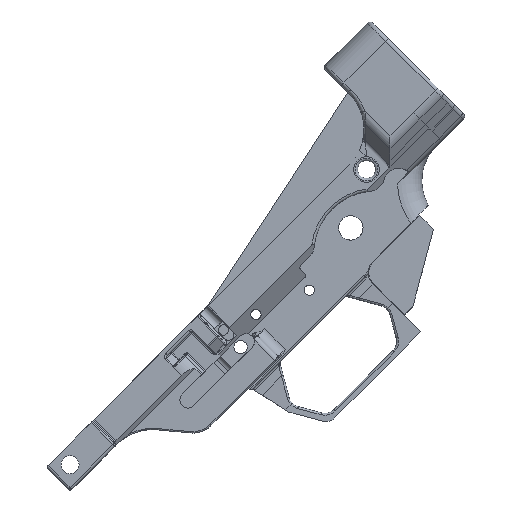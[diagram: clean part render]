
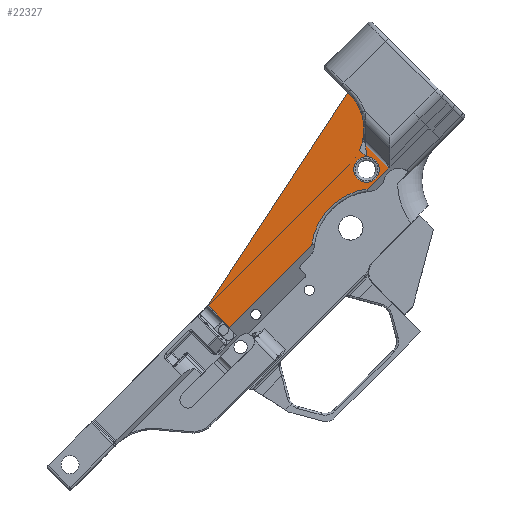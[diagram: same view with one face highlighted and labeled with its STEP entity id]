
A CAD part, front view. The second image highlights one B-rep face of the part: STEP entity #22327.
In plain terms, the highlighted planar face has unit normal (0, -1, 0).
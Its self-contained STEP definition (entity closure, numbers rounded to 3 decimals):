
#5577=CARTESIAN_POINT('',(-25.441,-18.567,22.339));
#5578=VERTEX_POINT('',#5577);
#5586=CARTESIAN_POINT('',(29.722,-18.567,77.502));
#5587=VERTEX_POINT('',#5586);
#5588=CARTESIAN_POINT('',(29.722,-18.567,77.502));
#5589=DIRECTION('',(-0.707,0.0,-0.707));
#5590=VECTOR('',#5589,78.013);
#5591=LINE('',#5588,#5590);
#5592=EDGE_CURVE('',#5587,#5578,#5591,.T.);
#8975=CARTESIAN_POINT('',(45.024,-18.567,76.019));
#8976=VERTEX_POINT('',#8975);
#8983=CARTESIAN_POINT('',(36.922,-18.567,67.916));
#8984=VERTEX_POINT('',#8983);
#8985=CARTESIAN_POINT('',(45.024,-18.567,76.019));
#8986=DIRECTION('',(-0.707,0.,-0.707));
#8987=VECTOR('',#8986,11.459);
#8988=LINE('',#8985,#8987);
#8989=EDGE_CURVE('',#8976,#8984,#8988,.T.);
#10142=CARTESIAN_POINT('',(41.289,-18.567,75.425));
#10143=VERTEX_POINT('',#10142);
#10144=CARTESIAN_POINT('',(36.289,-18.567,75.425));
#10145=DIRECTION('',(0.0,-1.0,0.0));
#10146=DIRECTION('',(1.0,0.0,0.0));
#10147=AXIS2_PLACEMENT_3D('',#10144,#10145,#10146);
#10148=CIRCLE('',#10147,5.);
#10149=EDGE_CURVE('',#10143,#10143,#10148,.T.);
#10159=CARTESIAN_POINT('',(29.013,-18.567,105.505));
#10160=VERTEX_POINT('',#10159);
#10161=CARTESIAN_POINT('',(35.207,-18.567,88.44));
#10162=VERTEX_POINT('',#10161);
#10163=CARTESIAN_POINT('',(16.079,-18.567,91.154));
#10164=DIRECTION('',(0.0,1.0,0.0));
#10165=DIRECTION('',(1.0,0.0,0.0));
#10166=AXIS2_PLACEMENT_3D('',#10163,#10164,#10165);
#10167=CIRCLE('',#10166,19.32);
#10168=EDGE_CURVE('',#10160,#10162,#10167,.T.);
#22223=CARTESIAN_POINT('',(-58.932,-18.567,-27.938));
#22224=DIRECTION('',(0.0,1.0,0.0));
#22225=DIRECTION('',(0.0,0.0,1.0));
#22226=AXIS2_PLACEMENT_3D('',#22223,#22224,#22225);
#22227=PLANE('',#22226);
#22228=ORIENTED_EDGE('',*,*,#8989,.F.);
#22229=CARTESIAN_POINT('',(35.986,-18.567,85.057));
#22230=VERTEX_POINT('',#22229);
#22231=CARTESIAN_POINT('',(45.024,-18.567,76.019));
#22232=DIRECTION('',(-0.707,0.0,0.707));
#22233=VECTOR('',#22232,12.782);
#22234=LINE('',#22231,#22233);
#22235=EDGE_CURVE('',#8976,#22230,#22234,.T.);
#22236=ORIENTED_EDGE('',*,*,#22235,.T.);
#22237=CARTESIAN_POINT('',(35.234,-18.567,87.194));
#22238=VERTEX_POINT('',#22237);
#22239=CARTESIAN_POINT('',(35.986,-18.567,85.057));
#22240=CARTESIAN_POINT('',(35.917,-18.567,85.232));
#22241=CARTESIAN_POINT('',(35.845,-18.566,85.408));
#22242=CARTESIAN_POINT('',(35.775,-18.566,85.583));
#22243=CARTESIAN_POINT('',(35.713,-18.566,85.735));
#22244=CARTESIAN_POINT('',(35.652,-18.567,85.886));
#22245=CARTESIAN_POINT('',(35.594,-18.567,86.04));
#22246=CARTESIAN_POINT('',(35.585,-18.567,86.063));
#22247=CARTESIAN_POINT('',(35.576,-18.567,86.087));
#22248=CARTESIAN_POINT('',(35.567,-18.567,86.11));
#22249=CARTESIAN_POINT('',(35.434,-18.567,86.464));
#22250=CARTESIAN_POINT('',(35.312,-18.567,86.821));
#22251=CARTESIAN_POINT('',(35.234,-18.567,87.194));
#22252=B_SPLINE_CURVE_WITH_KNOTS('',3,(#22239,#22240,#22241,#22242,#22243,#22244,#22245,#22246,#22247,#22248,#22249,#22250,#22251),.UNSPECIFIED.,.F.,.U.,(4,3,3,3,4),(-0.002,-0.002,-0.001,-0.001,0.0),.UNSPECIFIED.);
#22253=EDGE_CURVE('',#22230,#22238,#22252,.T.);
#22254=ORIENTED_EDGE('',*,*,#22253,.T.);
#22255=CARTESIAN_POINT('',(35.234,-18.567,87.194));
#22256=CARTESIAN_POINT('',(35.192,-18.567,87.398));
#22257=CARTESIAN_POINT('',(35.171,-18.567,87.608));
#22258=CARTESIAN_POINT('',(35.164,-18.567,88.024));
#22259=CARTESIAN_POINT('',(35.178,-18.567,88.234));
#22260=CARTESIAN_POINT('',(35.207,-18.567,88.44));
#22261=B_SPLINE_CURVE_WITH_KNOTS('',3,(#22255,#22256,#22257,#22258,#22259,#22260),.UNSPECIFIED.,.F.,.U.,(4,2,4),(-0.125,-0.062,0.),.UNSPECIFIED.);
#22262=EDGE_CURVE('',#22238,#10162,#22261,.T.);
#22263=ORIENTED_EDGE('',*,*,#22262,.T.);
#22264=ORIENTED_EDGE('',*,*,#10168,.F.);
#22265=CARTESIAN_POINT('',(29.722,-18.567,104.797));
#22266=VERTEX_POINT('',#22265);
#22267=CARTESIAN_POINT('',(29.013,-18.567,105.505));
#22268=DIRECTION('',(0.707,0.0,-0.707));
#22269=VECTOR('',#22268,1.002);
#22270=LINE('',#22267,#22269);
#22271=EDGE_CURVE('',#10160,#22266,#22270,.T.);
#22272=ORIENTED_EDGE('',*,*,#22271,.T.);
#22273=CARTESIAN_POINT('',(16.075,-18.567,91.15));
#22274=DIRECTION('',(0.0,-1.0,0.0));
#22275=DIRECTION('',(-1.0,0.0,0.0));
#22276=AXIS2_PLACEMENT_3D('',#22273,#22274,#22275);
#22277=CIRCLE('',#22276,19.3);
#22278=EDGE_CURVE('',#5587,#22266,#22277,.T.);
#22279=ORIENTED_EDGE('',*,*,#22278,.F.);
#22280=ORIENTED_EDGE('',*,*,#5592,.T.);
#22281=CARTESIAN_POINT('',(-23.477,-18.567,20.375));
#22282=VERTEX_POINT('',#22281);
#22283=CARTESIAN_POINT('',(-23.477,-18.567,20.375));
#22284=DIRECTION('',(-0.707,0.0,0.707));
#22285=VECTOR('',#22284,2.778);
#22286=LINE('',#22283,#22285);
#22287=EDGE_CURVE('',#22282,#5578,#22286,.T.);
#22288=ORIENTED_EDGE('',*,*,#22287,.F.);
#22289=CARTESIAN_POINT('',(-23.502,-18.566,20.35));
#22290=VERTEX_POINT('',#22289);
#22291=CARTESIAN_POINT('',(-23.502,-18.566,20.35));
#22292=CARTESIAN_POINT('',(-23.493,-18.566,20.358));
#22293=CARTESIAN_POINT('',(-23.485,-18.567,20.367));
#22294=CARTESIAN_POINT('',(-23.477,-18.567,20.375));
#22295=B_SPLINE_CURVE_WITH_KNOTS('',3,(#22291,#22292,#22293,#22294),.UNSPECIFIED.,.F.,.U.,(4,4),(0.001,1.0),.UNSPECIFIED.);
#22296=EDGE_CURVE('',#22290,#22282,#22295,.T.);
#22297=ORIENTED_EDGE('',*,*,#22296,.F.);
#22298=CARTESIAN_POINT('',(-17.081,-18.567,13.914));
#22299=VERTEX_POINT('',#22298);
#22300=CARTESIAN_POINT('',(-17.081,-18.567,13.914));
#22301=CARTESIAN_POINT('',(-19.221,-18.567,16.059));
#22302=CARTESIAN_POINT('',(-21.361,-18.567,18.205));
#22303=CARTESIAN_POINT('',(-23.502,-18.567,20.35));
#22304=QUASI_UNIFORM_CURVE('',3,(#22300,#22301,#22302,#22303),.UNSPECIFIED.,.F.,.U.);
#22305=EDGE_CURVE('',#22299,#22290,#22304,.T.);
#22306=ORIENTED_EDGE('',*,*,#22305,.F.);
#22307=CARTESIAN_POINT('',(14.954,-18.567,45.948));
#22308=VERTEX_POINT('',#22307);
#22309=CARTESIAN_POINT('',(14.954,-18.567,45.948));
#22310=DIRECTION('',(-0.707,0.,-0.707));
#22311=VECTOR('',#22310,45.303);
#22312=LINE('',#22309,#22311);
#22313=EDGE_CURVE('',#22308,#22299,#22312,.T.);
#22314=ORIENTED_EDGE('',*,*,#22313,.F.);
#22315=CARTESIAN_POINT('',(40.004,-18.567,42.866));
#22316=DIRECTION('',(0.,-1.0,0.));
#22317=DIRECTION('',(-0.993,0.,0.122));
#22318=AXIS2_PLACEMENT_3D('',#22315,#22316,#22317);
#22319=CIRCLE('',#22318,25.239);
#22320=EDGE_CURVE('',#8984,#22308,#22319,.T.);
#22321=ORIENTED_EDGE('',*,*,#22320,.F.);
#22322=EDGE_LOOP('',(#22228,#22236,#22254,#22263,#22264,#22272,#22279,#22280,#22288,#22297,#22306,#22314,#22321));
#22323=FACE_OUTER_BOUND('',#22322,.T.);
#22324=ORIENTED_EDGE('',*,*,#10149,.F.);
#22325=EDGE_LOOP('',(#22324));
#22326=FACE_BOUND('',#22325,.T.);
#22327=ADVANCED_FACE('',(#22323,#22326),#22227,.F.);
